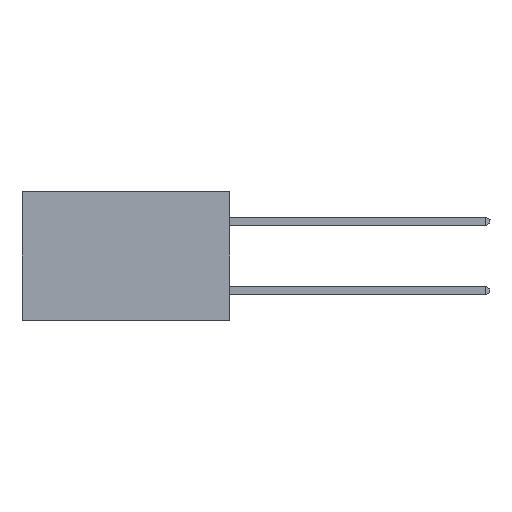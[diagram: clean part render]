
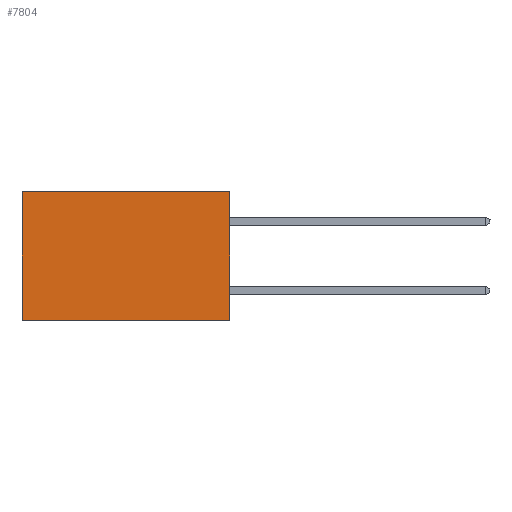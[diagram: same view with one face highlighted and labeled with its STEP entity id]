
A CAD part, left-side view. The second image highlights one B-rep face of the part: STEP entity #7804.
In plain terms, the highlighted planar face has unit normal (-1, 0, 0).
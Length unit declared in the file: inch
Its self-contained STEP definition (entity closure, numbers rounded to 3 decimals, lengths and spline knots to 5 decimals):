
#354 = DIRECTION ( 'NONE',  ( 1., 0., 0. ) ) ;
#470 = LINE ( 'NONE', #11795, #4804 ) ;
#589 = CARTESIAN_POINT ( 'NONE',  ( 0.298, 0., 0. ) ) ;
#610 = DIRECTION ( 'NONE',  ( 0., 1., 0. ) ) ;
#808 = EDGE_LOOP ( 'NONE', ( #10449, #4536, #13684, #985 ) ) ;
#985 = ORIENTED_EDGE ( 'NONE', *, *, #8708, .T. ) ;
#1630 = CARTESIAN_POINT ( 'NONE',  ( 0.298, 0., 0. ) ) ;
#1718 = VECTOR ( 'NONE', #12039, 39.37008 ) ;
#3174 = CARTESIAN_POINT ( 'NONE',  ( 0.298, 0., 0. ) ) ;
#3847 = CARTESIAN_POINT ( 'NONE',  ( 0.298, 0.6, -0.37 ) ) ;
#3972 = VECTOR ( 'NONE', #10378, 39.37008 ) ;
#4536 = ORIENTED_EDGE ( 'NONE', *, *, #10670, .F. ) ;
#4804 = VECTOR ( 'NONE', #610, 39.37008 ) ;
#5508 = EDGE_CURVE ( 'NONE', #8478, #10788, #9795, .T. ) ;
#5554 = VECTOR ( 'NONE', #15235, 39.37008 ) ;
#7282 = LINE ( 'NONE', #589, #3972 ) ;
#7692 = CARTESIAN_POINT ( 'NONE',  ( 0.298, 0.6, 0. ) ) ;
#7804 = ADVANCED_FACE ( 'NONE', ( #9166 ), #15372, .F. ) ;
#8190 = VERTEX_POINT ( 'NONE', #3174 ) ;
#8329 = LINE ( 'NONE', #1630, #1718 ) ;
#8478 = VERTEX_POINT ( 'NONE', #15835 ) ;
#8708 = EDGE_CURVE ( 'NONE', #8190, #8478, #8329, .T. ) ;
#9166 = FACE_OUTER_BOUND ( 'NONE', #808, .T. ) ;
#9795 = LINE ( 'NONE', #7692, #5554 ) ;
#10378 = DIRECTION ( 'NONE',  ( 0., 0., -1. ) ) ;
#10449 = ORIENTED_EDGE ( 'NONE', *, *, #5508, .T. ) ;
#10670 = EDGE_CURVE ( 'NONE', #11591, #10788, #470, .T. ) ;
#10788 = VERTEX_POINT ( 'NONE', #3847 ) ;
#11591 = VERTEX_POINT ( 'NONE', #14357 ) ;
#11697 = DIRECTION ( 'NONE',  ( 0., 0., -1. ) ) ;
#11795 = CARTESIAN_POINT ( 'NONE',  ( 0.298, 0., -0.37 ) ) ;
#12039 = DIRECTION ( 'NONE',  ( 0., 1., 0. ) ) ;
#12383 = EDGE_CURVE ( 'NONE', #8190, #11591, #7282, .T. ) ;
#13684 = ORIENTED_EDGE ( 'NONE', *, *, #12383, .F. ) ;
#14004 = AXIS2_PLACEMENT_3D ( 'NONE', #14171, #354, #11697 ) ;
#14171 = CARTESIAN_POINT ( 'NONE',  ( 0.298, 0., 0. ) ) ;
#14357 = CARTESIAN_POINT ( 'NONE',  ( 0.298, 0., -0.37 ) ) ;
#15235 = DIRECTION ( 'NONE',  ( 0., 0., -1. ) ) ;
#15372 = PLANE ( 'NONE',  #14004 ) ;
#15835 = CARTESIAN_POINT ( 'NONE',  ( 0.298, 0.6, 0. ) ) ;
